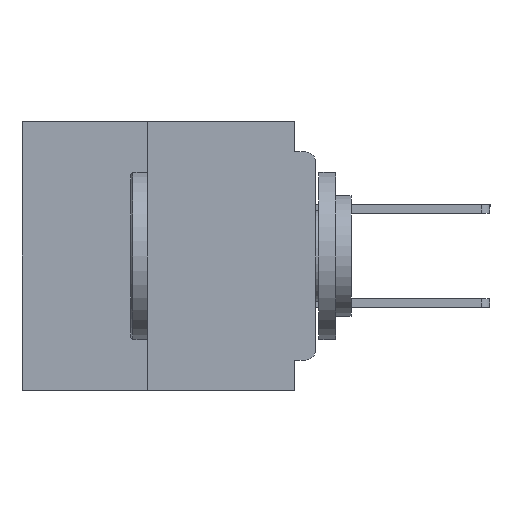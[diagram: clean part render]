
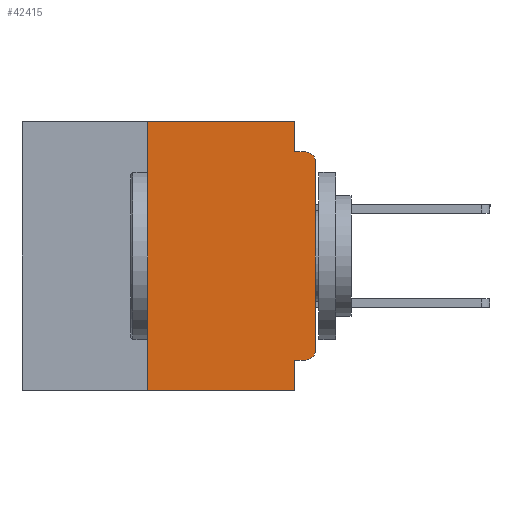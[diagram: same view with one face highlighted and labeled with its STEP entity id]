
A CAD part, left-side view. The second image highlights one B-rep face of the part: STEP entity #42415.
In plain terms, the highlighted planar face has unit normal (-1, 0, 0).
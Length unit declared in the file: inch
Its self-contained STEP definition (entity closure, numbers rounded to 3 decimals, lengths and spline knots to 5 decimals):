
#4 = CARTESIAN_POINT ( 'NONE',  ( 0., 0.437, 0. ) ) ;
#216 = CARTESIAN_POINT ( 'NONE',  ( 0., 0.031, 0. ) ) ;
#314 = EDGE_CURVE ( 'NONE', #46942, #47118, #25128, .T. ) ;
#729 = EDGE_CURVE ( 'NONE', #47118, #16447, #7823, .T. ) ;
#885 = VECTOR ( 'NONE', #46663, 39.37008 ) ;
#1639 = CARTESIAN_POINT ( 'NONE',  ( 0., 0.031, -0.355 ) ) ;
#1786 = DIRECTION ( 'NONE',  ( 0., -1., 0. ) ) ;
#1856 = VERTEX_POINT ( 'NONE', #1639 ) ;
#1980 = CARTESIAN_POINT ( 'NONE',  ( 0., 0.031, 0. ) ) ;
#2425 = VERTEX_POINT ( 'NONE', #26898 ) ;
#2663 = EDGE_CURVE ( 'NONE', #39664, #46942, #5275, .T. ) ;
#2674 = LINE ( 'NONE', #31338, #11453 ) ;
#2735 = LINE ( 'NONE', #28882, #40686 ) ;
#3075 = DIRECTION ( 'NONE',  ( 0., -1., 0. ) ) ;
#3319 = CARTESIAN_POINT ( 'NONE',  ( 0., 0.25, 0. ) ) ;
#3572 = VECTOR ( 'NONE', #15386, 39.37008 ) ;
#4022 = DIRECTION ( 'NONE',  ( 0., 0., -1. ) ) ;
#4259 = ORIENTED_EDGE ( 'NONE', *, *, #32258, .F. ) ;
#5275 = CIRCLE ( 'NONE', #25937, 0.015 ) ;
#6215 = AXIS2_PLACEMENT_3D ( 'NONE', #13965, #39483, #17639 ) ;
#6685 = ORIENTED_EDGE ( 'NONE', *, *, #9173, .F. ) ;
#7823 = CIRCLE ( 'NONE', #14253, 0.015 ) ;
#8133 = CARTESIAN_POINT ( 'NONE',  ( 0., 0., -0.34 ) ) ;
#8813 = ORIENTED_EDGE ( 'NONE', *, *, #37620, .T. ) ;
#9173 = EDGE_CURVE ( 'NONE', #13784, #16447, #2674, .T. ) ;
#9350 = CARTESIAN_POINT ( 'NONE',  ( 0., 0., 0. ) ) ;
#9757 = DIRECTION ( 'NONE',  ( 0., 0., 1. ) ) ;
#10223 = PLANE ( 'NONE',  #6215 ) ;
#10797 = EDGE_CURVE ( 'NONE', #18680, #18568, #37113, .T. ) ;
#11453 = VECTOR ( 'NONE', #1786, 39.37008 ) ;
#11617 = CARTESIAN_POINT ( 'NONE',  ( 0., 0., -0.355 ) ) ;
#12490 = CARTESIAN_POINT ( 'NONE',  ( 0., 0.015, -0.06 ) ) ;
#12933 = EDGE_CURVE ( 'NONE', #1856, #2425, #29221, .T. ) ;
#13390 = CARTESIAN_POINT ( 'NONE',  ( 0., 0.015, -0.045 ) ) ;
#13784 = VERTEX_POINT ( 'NONE', #22444 ) ;
#13965 = CARTESIAN_POINT ( 'NONE',  ( 0., 0.437, 0. ) ) ;
#14253 = AXIS2_PLACEMENT_3D ( 'NONE', #12490, #38834, #16385 ) ;
#14786 = ORIENTED_EDGE ( 'NONE', *, *, #314, .T. ) ;
#15082 = DIRECTION ( 'NONE',  ( 0., -1., 0. ) ) ;
#15386 = DIRECTION ( 'NONE',  ( 0., 1., 0. ) ) ;
#16385 = DIRECTION ( 'NONE',  ( 0., 0., -1. ) ) ;
#16447 = VERTEX_POINT ( 'NONE', #13390 ) ;
#17038 = DIRECTION ( 'NONE',  ( 0., 0., -1. ) ) ;
#17146 = DIRECTION ( 'NONE',  ( -1., 0., 0. ) ) ;
#17238 = CARTESIAN_POINT ( 'NONE',  ( 0., 0.015, -0.34 ) ) ;
#17639 = DIRECTION ( 'NONE',  ( 0., 0., -1. ) ) ;
#18408 = LINE ( 'NONE', #41871, #26953 ) ;
#18568 = VERTEX_POINT ( 'NONE', #1980 ) ;
#18641 = ORIENTED_EDGE ( 'NONE', *, *, #21168, .F. ) ;
#18680 = VERTEX_POINT ( 'NONE', #3319 ) ;
#19995 = ORIENTED_EDGE ( 'NONE', *, *, #729, .T. ) ;
#21168 = EDGE_CURVE ( 'NONE', #39664, #1856, #42588, .T. ) ;
#21254 = CARTESIAN_POINT ( 'NONE',  ( 0., 0.031, -0.4 ) ) ;
#22444 = CARTESIAN_POINT ( 'NONE',  ( 0., 0.031, -0.045 ) ) ;
#23843 = EDGE_CURVE ( 'NONE', #31902, #18680, #18408, .T. ) ;
#23912 = CARTESIAN_POINT ( 'NONE',  ( 0., 0., -0.06 ) ) ;
#25128 = LINE ( 'NONE', #9350, #43355 ) ;
#25937 = AXIS2_PLACEMENT_3D ( 'NONE', #17238, #17146, #17038 ) ;
#26888 = EDGE_LOOP ( 'NONE', ( #14786, #19995, #6685, #4259, #37617, #47531, #8813, #29390, #18641, #45995 ) ) ;
#26898 = CARTESIAN_POINT ( 'NONE',  ( 0., 0.031, -0.4 ) ) ;
#26953 = VECTOR ( 'NONE', #9757, 39.37008 ) ;
#27363 = LINE ( 'NONE', #216, #45582 ) ;
#27368 = CARTESIAN_POINT ( 'NONE',  ( 0., 0.015, -0.355 ) ) ;
#27446 = VECTOR ( 'NONE', #15082, 39.37008 ) ;
#28882 = CARTESIAN_POINT ( 'NONE',  ( 0., 0.437, -0.4 ) ) ;
#29221 = LINE ( 'NONE', #21254, #885 ) ;
#29390 = ORIENTED_EDGE ( 'NONE', *, *, #12933, .F. ) ;
#31338 = CARTESIAN_POINT ( 'NONE',  ( 0., 0., -0.045 ) ) ;
#31902 = VERTEX_POINT ( 'NONE', #41575 ) ;
#32258 = EDGE_CURVE ( 'NONE', #18568, #13784, #27363, .T. ) ;
#37113 = LINE ( 'NONE', #4, #27446 ) ;
#37617 = ORIENTED_EDGE ( 'NONE', *, *, #10797, .F. ) ;
#37620 = EDGE_CURVE ( 'NONE', #31902, #2425, #2735, .T. ) ;
#37990 = DIRECTION ( 'NONE',  ( 0., 0., 1. ) ) ;
#38834 = DIRECTION ( 'NONE',  ( -1., 0., 0. ) ) ;
#39483 = DIRECTION ( 'NONE',  ( 1., 0., 0. ) ) ;
#39664 = VERTEX_POINT ( 'NONE', #27368 ) ;
#40686 = VECTOR ( 'NONE', #3075, 39.37008 ) ;
#41575 = CARTESIAN_POINT ( 'NONE',  ( 0., 0.25, -0.4 ) ) ;
#41871 = CARTESIAN_POINT ( 'NONE',  ( 0., 0.25, -0.4 ) ) ;
#42415 = ADVANCED_FACE ( 'NONE', ( #47075 ), #10223, .F. ) ;
#42588 = LINE ( 'NONE', #11617, #3572 ) ;
#43355 = VECTOR ( 'NONE', #37990, 39.37008 ) ;
#45582 = VECTOR ( 'NONE', #4022, 39.37008 ) ;
#45995 = ORIENTED_EDGE ( 'NONE', *, *, #2663, .T. ) ;
#46663 = DIRECTION ( 'NONE',  ( 0., 0., -1. ) ) ;
#46942 = VERTEX_POINT ( 'NONE', #8133 ) ;
#47075 = FACE_OUTER_BOUND ( 'NONE', #26888, .T. ) ;
#47118 = VERTEX_POINT ( 'NONE', #23912 ) ;
#47531 = ORIENTED_EDGE ( 'NONE', *, *, #23843, .F. ) ;
